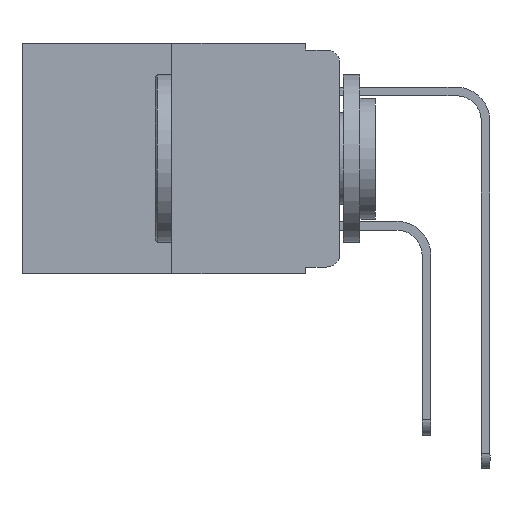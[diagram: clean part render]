
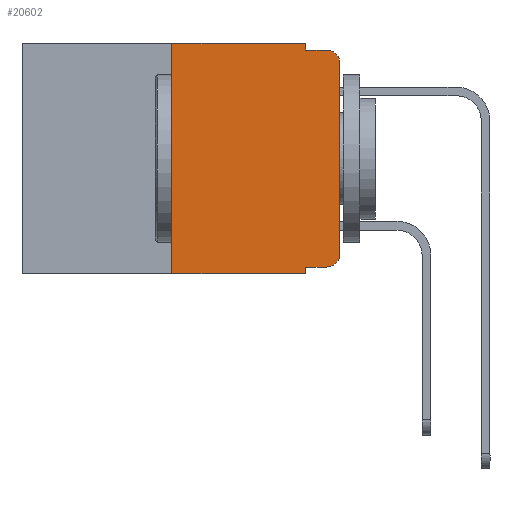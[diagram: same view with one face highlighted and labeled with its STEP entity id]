
A CAD part, left-side view. The second image highlights one B-rep face of the part: STEP entity #20602.
In plain terms, the highlighted planar face has unit normal (-1, 0, 0).
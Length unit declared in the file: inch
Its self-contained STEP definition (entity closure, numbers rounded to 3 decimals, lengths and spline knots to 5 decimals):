
#912 = VERTEX_POINT ( 'NONE', #21205 ) ;
#1138 = CARTESIAN_POINT ( 'NONE',  ( 0., 0., 0. ) ) ;
#1603 = VERTEX_POINT ( 'NONE', #22152 ) ;
#1673 = DIRECTION ( 'NONE',  ( -1., 0., 0. ) ) ;
#1877 = EDGE_CURVE ( 'NONE', #12268, #10832, #19281, .T. ) ;
#2653 = CIRCLE ( 'NONE', #7426, 0.02 ) ;
#2817 = ORIENTED_EDGE ( 'NONE', *, *, #15147, .T. ) ;
#2829 = DIRECTION ( 'NONE',  ( 0., 0., -1. ) ) ;
#3225 = EDGE_CURVE ( 'NONE', #10832, #21262, #12217, .T. ) ;
#3319 = EDGE_CURVE ( 'NONE', #12274, #13050, #6993, .T. ) ;
#4250 = ORIENTED_EDGE ( 'NONE', *, *, #3319, .T. ) ;
#4369 = VECTOR ( 'NONE', #14328, 39.37008 ) ;
#4395 = FACE_OUTER_BOUND ( 'NONE', #13522, .T. ) ;
#4528 = LINE ( 'NONE', #14093, #13268 ) ;
#4665 = ORIENTED_EDGE ( 'NONE', *, *, #3225, .F. ) ;
#4860 = ORIENTED_EDGE ( 'NONE', *, *, #16116, .T. ) ;
#5124 = DIRECTION ( 'NONE',  ( 0., 0., 1. ) ) ;
#5131 = DIRECTION ( 'NONE',  ( 0., -1., 0. ) ) ;
#5845 = ORIENTED_EDGE ( 'NONE', *, *, #9805, .T. ) ;
#5866 = CARTESIAN_POINT ( 'NONE',  ( 0., 0.051, -0.333 ) ) ;
#5991 = DIRECTION ( 'NONE',  ( 0., -1., 0. ) ) ;
#6044 = CARTESIAN_POINT ( 'NONE',  ( 0., 0.051, -0.343 ) ) ;
#6134 = DIRECTION ( 'NONE',  ( 0., 0., -1. ) ) ;
#6558 = CARTESIAN_POINT ( 'NONE',  ( 0., 0.051, 0. ) ) ;
#6760 = LINE ( 'NONE', #17814, #4369 ) ;
#6960 = CARTESIAN_POINT ( 'NONE',  ( 0., 0.051, -0.01 ) ) ;
#6993 = LINE ( 'NONE', #1138, #18518 ) ;
#7426 = AXIS2_PLACEMENT_3D ( 'NONE', #18700, #1673, #13239 ) ;
#7515 = ORIENTED_EDGE ( 'NONE', *, *, #15153, .F. ) ;
#8196 = AXIS2_PLACEMENT_3D ( 'NONE', #18945, #17799, #22791 ) ;
#8487 = DIRECTION ( 'NONE',  ( 0., -1., 0. ) ) ;
#8612 = LINE ( 'NONE', #10591, #9912 ) ;
#9329 = CARTESIAN_POINT ( 'NONE',  ( 0., 0., -0.313 ) ) ;
#9805 = EDGE_CURVE ( 'NONE', #13220, #12274, #14535, .T. ) ;
#9867 = CARTESIAN_POINT ( 'NONE',  ( 0., 0.051, 0. ) ) ;
#9912 = VECTOR ( 'NONE', #5131, 39.37008 ) ;
#10344 = CARTESIAN_POINT ( 'NONE',  ( 0., 0.473, 0. ) ) ;
#10460 = DIRECTION ( 'NONE',  ( 1., 0., 0. ) ) ;
#10591 = CARTESIAN_POINT ( 'NONE',  ( 0., 0.473, -0.343 ) ) ;
#10832 = VERTEX_POINT ( 'NONE', #6558 ) ;
#11008 = CARTESIAN_POINT ( 'NONE',  ( 0., 0., -0.03 ) ) ;
#11060 = EDGE_CURVE ( 'NONE', #13050, #1603, #2653, .T. ) ;
#11572 = LINE ( 'NONE', #5866, #13523 ) ;
#12007 = ORIENTED_EDGE ( 'NONE', *, *, #1877, .F. ) ;
#12217 = LINE ( 'NONE', #9867, #19312 ) ;
#12268 = VERTEX_POINT ( 'NONE', #22621 ) ;
#12274 = VERTEX_POINT ( 'NONE', #9329 ) ;
#12851 = ORIENTED_EDGE ( 'NONE', *, *, #20229, .F. ) ;
#12877 = AXIS2_PLACEMENT_3D ( 'NONE', #10344, #10460, #18032 ) ;
#13050 = VERTEX_POINT ( 'NONE', #11008 ) ;
#13220 = VERTEX_POINT ( 'NONE', #13867 ) ;
#13239 = DIRECTION ( 'NONE',  ( 0., 0., -1. ) ) ;
#13268 = VECTOR ( 'NONE', #21662, 39.37008 ) ;
#13522 = EDGE_LOOP ( 'NONE', ( #4250, #15725, #7515, #4665, #12007, #12851, #2817, #15969, #4860, #5845 ) ) ;
#13523 = VECTOR ( 'NONE', #5991, 39.37008 ) ;
#13867 = CARTESIAN_POINT ( 'NONE',  ( 0., 0.02, -0.333 ) ) ;
#14093 = CARTESIAN_POINT ( 'NONE',  ( 0., 0.25, 0. ) ) ;
#14328 = DIRECTION ( 'NONE',  ( 0., -1., 0. ) ) ;
#14482 = VERTEX_POINT ( 'NONE', #6044 ) ;
#14535 = CIRCLE ( 'NONE', #8196, 0.02 ) ;
#15147 = EDGE_CURVE ( 'NONE', #23675, #14482, #8612, .T. ) ;
#15153 = EDGE_CURVE ( 'NONE', #21262, #1603, #6760, .T. ) ;
#15725 = ORIENTED_EDGE ( 'NONE', *, *, #11060, .T. ) ;
#15969 = ORIENTED_EDGE ( 'NONE', *, *, #16661, .F. ) ;
#16116 = EDGE_CURVE ( 'NONE', #912, #13220, #11572, .T. ) ;
#16120 = LINE ( 'NONE', #17755, #21451 ) ;
#16661 = EDGE_CURVE ( 'NONE', #912, #14482, #16120, .T. ) ;
#17755 = CARTESIAN_POINT ( 'NONE',  ( 0., 0.051, 0. ) ) ;
#17799 = DIRECTION ( 'NONE',  ( -1., 0., 0. ) ) ;
#17803 = CARTESIAN_POINT ( 'NONE',  ( 0., 0.473, 0. ) ) ;
#17814 = CARTESIAN_POINT ( 'NONE',  ( 0., 0.051, -0.01 ) ) ;
#18032 = DIRECTION ( 'NONE',  ( 0., 0., -1. ) ) ;
#18518 = VECTOR ( 'NONE', #5124, 39.37008 ) ;
#18700 = CARTESIAN_POINT ( 'NONE',  ( 0., 0.02, -0.03 ) ) ;
#18945 = CARTESIAN_POINT ( 'NONE',  ( 0., 0.02, -0.313 ) ) ;
#19281 = LINE ( 'NONE', #17803, #20770 ) ;
#19312 = VECTOR ( 'NONE', #6134, 39.37008 ) ;
#20229 = EDGE_CURVE ( 'NONE', #23675, #12268, #4528, .T. ) ;
#20602 = ADVANCED_FACE ( 'NONE', ( #4395 ), #23499, .F. ) ;
#20770 = VECTOR ( 'NONE', #8487, 39.37008 ) ;
#21205 = CARTESIAN_POINT ( 'NONE',  ( 0., 0.051, -0.333 ) ) ;
#21262 = VERTEX_POINT ( 'NONE', #6960 ) ;
#21451 = VECTOR ( 'NONE', #2829, 39.37008 ) ;
#21662 = DIRECTION ( 'NONE',  ( 0., 0., 1. ) ) ;
#22152 = CARTESIAN_POINT ( 'NONE',  ( 0., 0.02, -0.01 ) ) ;
#22621 = CARTESIAN_POINT ( 'NONE',  ( 0., 0.25, 0. ) ) ;
#22648 = CARTESIAN_POINT ( 'NONE',  ( 0., 0.25, -0.343 ) ) ;
#22791 = DIRECTION ( 'NONE',  ( 0., 0., -1. ) ) ;
#23499 = PLANE ( 'NONE',  #12877 ) ;
#23675 = VERTEX_POINT ( 'NONE', #22648 ) ;
